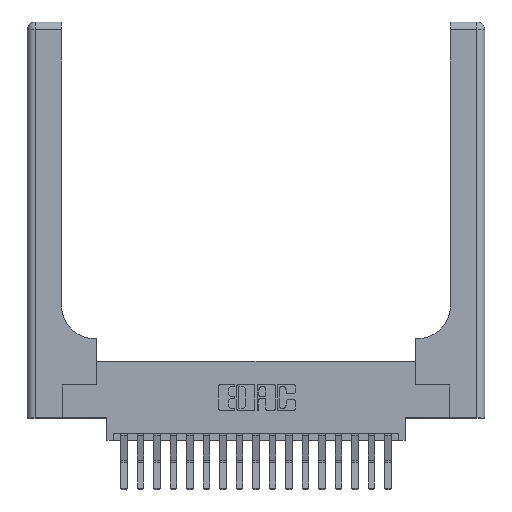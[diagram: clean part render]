
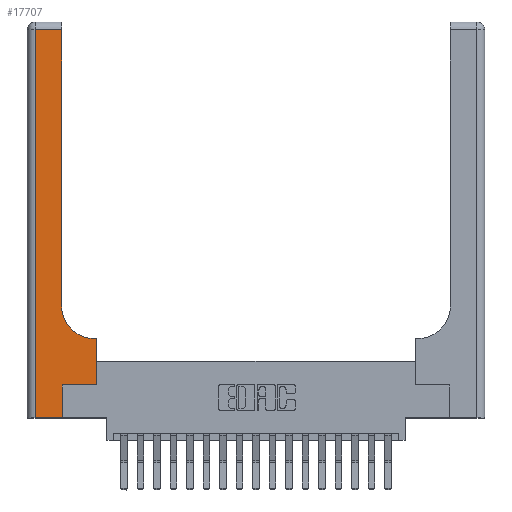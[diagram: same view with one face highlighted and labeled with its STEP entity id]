
A CAD part, top view. The second image highlights one B-rep face of the part: STEP entity #17707.
In plain terms, the highlighted planar face has unit normal (0, 0, 1).
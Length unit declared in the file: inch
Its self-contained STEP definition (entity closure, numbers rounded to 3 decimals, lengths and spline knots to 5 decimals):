
#52 = ORIENTED_EDGE ( 'NONE', *, *, #6622, .T. ) ;
#87 = CARTESIAN_POINT ( 'NONE',  ( 0.06, 2.94, 0.37 ) ) ;
#290 = DIRECTION ( 'NONE',  ( 0., 1., 0. ) ) ;
#523 = VERTEX_POINT ( 'NONE', #4947 ) ;
#530 = ORIENTED_EDGE ( 'NONE', *, *, #5419, .T. ) ;
#677 = CIRCLE ( 'NONE', #8719, 0.25 ) ;
#883 = CARTESIAN_POINT ( 'NONE',  ( 0., 3., 0.37 ) ) ;
#1104 = VERTEX_POINT ( 'NONE', #5894 ) ;
#1297 = EDGE_CURVE ( 'NONE', #1104, #6447, #1421, .T. ) ;
#1382 = CARTESIAN_POINT ( 'NONE',  ( 0., 0., 0.37 ) ) ;
#1421 = LINE ( 'NONE', #14137, #17310 ) ;
#1509 = VECTOR ( 'NONE', #12150, 39.37008 ) ;
#1921 = CARTESIAN_POINT ( 'NONE',  ( 0.528, 0.25, 0.37 ) ) ;
#2119 = DIRECTION ( 'NONE',  ( 0., 0., -1. ) ) ;
#2122 = CARTESIAN_POINT ( 'NONE',  ( 0.26, 0.85, 0.37 ) ) ;
#2208 = ORIENTED_EDGE ( 'NONE', *, *, #9372, .T. ) ;
#3045 = VECTOR ( 'NONE', #16470, 39.37008 ) ;
#3163 = ORIENTED_EDGE ( 'NONE', *, *, #14535, .T. ) ;
#3444 = DIRECTION ( 'NONE',  ( 0., 1., 0. ) ) ;
#3942 = DIRECTION ( 'NONE',  ( -1., 0., 0. ) ) ;
#4588 = ORIENTED_EDGE ( 'NONE', *, *, #7995, .T. ) ;
#4762 = CARTESIAN_POINT ( 'NONE',  ( 0.528, 0.6, 0.37 ) ) ;
#4767 = CARTESIAN_POINT ( 'NONE',  ( 0.51, 0.6, 0.37 ) ) ;
#4877 = CARTESIAN_POINT ( 'NONE',  ( 0.265, 0.25, 0.37 ) ) ;
#4947 = CARTESIAN_POINT ( 'NONE',  ( 0.06, 0., 0.37 ) ) ;
#5419 = EDGE_CURVE ( 'NONE', #8399, #14732, #11332, .T. ) ;
#5526 = DIRECTION ( 'NONE',  ( -1., 0., 0. ) ) ;
#5894 = CARTESIAN_POINT ( 'NONE',  ( 0.265, 0., 0.37 ) ) ;
#6009 = VERTEX_POINT ( 'NONE', #6843 ) ;
#6447 = VERTEX_POINT ( 'NONE', #4877 ) ;
#6477 = CARTESIAN_POINT ( 'NONE',  ( 0.06, 3., 0.37 ) ) ;
#6544 = DIRECTION ( 'NONE',  ( 0., -1., 0. ) ) ;
#6622 = EDGE_CURVE ( 'NONE', #6447, #9983, #9362, .T. ) ;
#6843 = CARTESIAN_POINT ( 'NONE',  ( 0.26, 2.94, 0.37 ) ) ;
#7213 = VECTOR ( 'NONE', #5526, 39.37008 ) ;
#7572 = LINE ( 'NONE', #10322, #3045 ) ;
#7677 = EDGE_CURVE ( 'NONE', #9983, #8399, #8590, .T. ) ;
#7995 = EDGE_CURVE ( 'NONE', #14732, #9807, #677, .T. ) ;
#8012 = DIRECTION ( 'NONE',  ( -1., 0., 0. ) ) ;
#8263 = LINE ( 'NONE', #6477, #11894 ) ;
#8399 = VERTEX_POINT ( 'NONE', #4762 ) ;
#8590 = LINE ( 'NONE', #1921, #16335 ) ;
#8719 = AXIS2_PLACEMENT_3D ( 'NONE', #11305, #2119, #12937 ) ;
#9362 = LINE ( 'NONE', #12994, #17108 ) ;
#9372 = EDGE_CURVE ( 'NONE', #9807, #6009, #7572, .T. ) ;
#9807 = VERTEX_POINT ( 'NONE', #2122 ) ;
#9983 = VERTEX_POINT ( 'NONE', #17789 ) ;
#10077 = PLANE ( 'NONE',  #18476 ) ;
#10296 = VERTEX_POINT ( 'NONE', #87 ) ;
#10322 = CARTESIAN_POINT ( 'NONE',  ( 0.26, 3., 0.37 ) ) ;
#11305 = CARTESIAN_POINT ( 'NONE',  ( 0.51, 0.85, 0.37 ) ) ;
#11332 = LINE ( 'NONE', #19395, #7213 ) ;
#11825 = ORIENTED_EDGE ( 'NONE', *, *, #1297, .T. ) ;
#11894 = VECTOR ( 'NONE', #6544, 39.37008 ) ;
#12150 = DIRECTION ( 'NONE',  ( 1., 0., 0. ) ) ;
#12455 = EDGE_CURVE ( 'NONE', #10296, #523, #8263, .T. ) ;
#12937 = DIRECTION ( 'NONE',  ( 1., 0., 0. ) ) ;
#12983 = VECTOR ( 'NONE', #8012, 39.37008 ) ;
#12994 = CARTESIAN_POINT ( 'NONE',  ( 0.265, 0.25, 0.37 ) ) ;
#13252 = DIRECTION ( 'NONE',  ( 0., 0., -1. ) ) ;
#13843 = LINE ( 'NONE', #1382, #1509 ) ;
#14137 = CARTESIAN_POINT ( 'NONE',  ( 0.265, 0., 0.37 ) ) ;
#14339 = EDGE_LOOP ( 'NONE', ( #2208, #18568, #15022, #3163, #11825, #52, #16427, #530, #4588 ) ) ;
#14535 = EDGE_CURVE ( 'NONE', #523, #1104, #13843, .T. ) ;
#14732 = VERTEX_POINT ( 'NONE', #4767 ) ;
#15022 = ORIENTED_EDGE ( 'NONE', *, *, #12455, .T. ) ;
#16038 = DIRECTION ( 'NONE',  ( 1., 0., 0. ) ) ;
#16054 = LINE ( 'NONE', #17267, #12983 ) ;
#16335 = VECTOR ( 'NONE', #3444, 39.37008 ) ;
#16427 = ORIENTED_EDGE ( 'NONE', *, *, #7677, .T. ) ;
#16470 = DIRECTION ( 'NONE',  ( 0., 1., 0. ) ) ;
#17108 = VECTOR ( 'NONE', #16038, 39.37008 ) ;
#17267 = CARTESIAN_POINT ( 'NONE',  ( 0., 2.94, 0.37 ) ) ;
#17310 = VECTOR ( 'NONE', #290, 39.37008 ) ;
#17707 = ADVANCED_FACE ( 'NONE', ( #19176 ), #10077, .F. ) ;
#17789 = CARTESIAN_POINT ( 'NONE',  ( 0.528, 0.25, 0.37 ) ) ;
#18476 = AXIS2_PLACEMENT_3D ( 'NONE', #883, #13252, #3942 ) ;
#18568 = ORIENTED_EDGE ( 'NONE', *, *, #18711, .T. ) ;
#18711 = EDGE_CURVE ( 'NONE', #6009, #10296, #16054, .T. ) ;
#19176 = FACE_OUTER_BOUND ( 'NONE', #14339, .T. ) ;
#19395 = CARTESIAN_POINT ( 'NONE',  ( 0.26, 0.6, 0.37 ) ) ;
